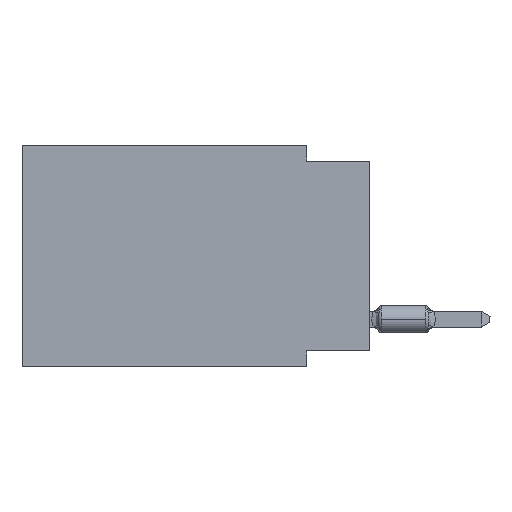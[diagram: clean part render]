
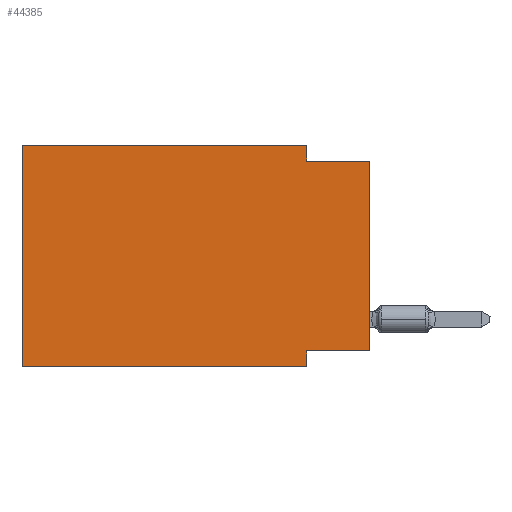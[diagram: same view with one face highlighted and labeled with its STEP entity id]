
A CAD part, left-side view. The second image highlights one B-rep face of the part: STEP entity #44385.
In plain terms, the highlighted planar face has unit normal (-1, 0, 0).
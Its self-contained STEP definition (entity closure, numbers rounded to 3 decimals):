
#2162 = CARTESIAN_POINT ( 'NONE',  ( 0., 0., 0. ) ) ;
#3360 = DIRECTION ( 'NONE',  ( 0., 0., -1. ) ) ;
#4715 = VECTOR ( 'NONE', #23454, 1000. ) ;
#4883 = CARTESIAN_POINT ( 'NONE',  ( 0., 13.97, 0. ) ) ;
#5996 = VECTOR ( 'NONE', #67099, 1000. ) ;
#6392 = VERTEX_POINT ( 'NONE', #4883 ) ;
#6437 = VECTOR ( 'NONE', #41418, 1000. ) ;
#6878 = CARTESIAN_POINT ( 'NONE',  ( 0., 2.54, 0. ) ) ;
#9310 = DIRECTION ( 'NONE',  ( 1., 0., 0. ) ) ;
#9572 = EDGE_CURVE ( 'NONE', #57525, #40581, #71930, .T. ) ;
#9703 = LINE ( 'NONE', #2162, #32992 ) ;
#10266 = CARTESIAN_POINT ( 'NONE',  ( 0., 2.54, -8.89 ) ) ;
#10816 = AXIS2_PLACEMENT_3D ( 'NONE', #15267, #9310, #3360 ) ;
#11022 = EDGE_CURVE ( 'NONE', #37612, #57525, #23970, .T. ) ;
#11698 = VERTEX_POINT ( 'NONE', #35284 ) ;
#13405 = VECTOR ( 'NONE', #28536, 1000. ) ;
#14167 = DIRECTION ( 'NONE',  ( 0., 1., 0. ) ) ;
#15267 = CARTESIAN_POINT ( 'NONE',  ( 0., 13.97, 0. ) ) ;
#16076 = ORIENTED_EDGE ( 'NONE', *, *, #9572, .F. ) ;
#17037 = LINE ( 'NONE', #28922, #13405 ) ;
#17757 = VECTOR ( 'NONE', #39141, 1000. ) ;
#19483 = ORIENTED_EDGE ( 'NONE', *, *, #60723, .F. ) ;
#20912 = CARTESIAN_POINT ( 'NONE',  ( 0., 0., -8.255 ) ) ;
#21453 = CARTESIAN_POINT ( 'NONE',  ( 0., 0., -8.255 ) ) ;
#23318 = ORIENTED_EDGE ( 'NONE', *, *, #60796, .F. ) ;
#23454 = DIRECTION ( 'NONE',  ( 0., -1., 0. ) ) ;
#23970 = LINE ( 'NONE', #6878, #74959 ) ;
#28536 = DIRECTION ( 'NONE',  ( 0., 0., 1. ) ) ;
#28922 = CARTESIAN_POINT ( 'NONE',  ( 0., 13.97, 0. ) ) ;
#30836 = LINE ( 'NONE', #20912, #45583 ) ;
#30852 = ORIENTED_EDGE ( 'NONE', *, *, #55904, .F. ) ;
#31834 = DIRECTION ( 'NONE',  ( 0., 0., -1. ) ) ;
#32680 = DIRECTION ( 'NONE',  ( 0., 0., 1. ) ) ;
#32745 = ORIENTED_EDGE ( 'NONE', *, *, #33729, .T. ) ;
#32992 = VECTOR ( 'NONE', #32680, 1000. ) ;
#33447 = EDGE_CURVE ( 'NONE', #6392, #37612, #62702, .T. ) ;
#33729 = EDGE_CURVE ( 'NONE', #11698, #37311, #35337, .T. ) ;
#35284 = CARTESIAN_POINT ( 'NONE',  ( 0., 13.97, -8.89 ) ) ;
#35337 = LINE ( 'NONE', #65471, #4715 ) ;
#37311 = VERTEX_POINT ( 'NONE', #10266 ) ;
#37612 = VERTEX_POINT ( 'NONE', #52954 ) ;
#37746 = CARTESIAN_POINT ( 'NONE',  ( 0., 13.97, 0. ) ) ;
#39141 = DIRECTION ( 'NONE',  ( 0., 0., -1. ) ) ;
#39519 = LINE ( 'NONE', #44679, #17757 ) ;
#40581 = VERTEX_POINT ( 'NONE', #51992 ) ;
#41418 = DIRECTION ( 'NONE',  ( 0., -1., 0. ) ) ;
#44385 = ADVANCED_FACE ( 'NONE', ( #45391 ), #69566, .F. ) ;
#44679 = CARTESIAN_POINT ( 'NONE',  ( 0., 2.54, -8.89 ) ) ;
#45391 = FACE_OUTER_BOUND ( 'NONE', #63770, .T. ) ;
#45583 = VECTOR ( 'NONE', #14167, 1000. ) ;
#48462 = EDGE_CURVE ( 'NONE', #53333, #40581, #9703, .T. ) ;
#50587 = VERTEX_POINT ( 'NONE', #69857 ) ;
#51992 = CARTESIAN_POINT ( 'NONE',  ( 0., 0., -0.635 ) ) ;
#52954 = CARTESIAN_POINT ( 'NONE',  ( 0., 2.54, 0. ) ) ;
#53333 = VERTEX_POINT ( 'NONE', #21453 ) ;
#55904 = EDGE_CURVE ( 'NONE', #11698, #6392, #17037, .T. ) ;
#57525 = VERTEX_POINT ( 'NONE', #75624 ) ;
#57852 = ORIENTED_EDGE ( 'NONE', *, *, #48462, .T. ) ;
#60723 = EDGE_CURVE ( 'NONE', #53333, #50587, #30836, .T. ) ;
#60796 = EDGE_CURVE ( 'NONE', #50587, #37311, #39519, .T. ) ;
#62702 = LINE ( 'NONE', #37746, #5996 ) ;
#63770 = EDGE_LOOP ( 'NONE', ( #57852, #16076, #74216, #76051, #30852, #32745, #23318, #19483 ) ) ;
#65471 = CARTESIAN_POINT ( 'NONE',  ( 0., 13.97, -8.89 ) ) ;
#67099 = DIRECTION ( 'NONE',  ( 0., -1., 0. ) ) ;
#67146 = CARTESIAN_POINT ( 'NONE',  ( 0., 0., -0.635 ) ) ;
#69566 = PLANE ( 'NONE',  #10816 ) ;
#69857 = CARTESIAN_POINT ( 'NONE',  ( 0., 2.54, -8.255 ) ) ;
#71930 = LINE ( 'NONE', #67146, #6437 ) ;
#74216 = ORIENTED_EDGE ( 'NONE', *, *, #11022, .F. ) ;
#74959 = VECTOR ( 'NONE', #31834, 1000. ) ;
#75624 = CARTESIAN_POINT ( 'NONE',  ( 0., 2.54, -0.635 ) ) ;
#76051 = ORIENTED_EDGE ( 'NONE', *, *, #33447, .F. ) ;
